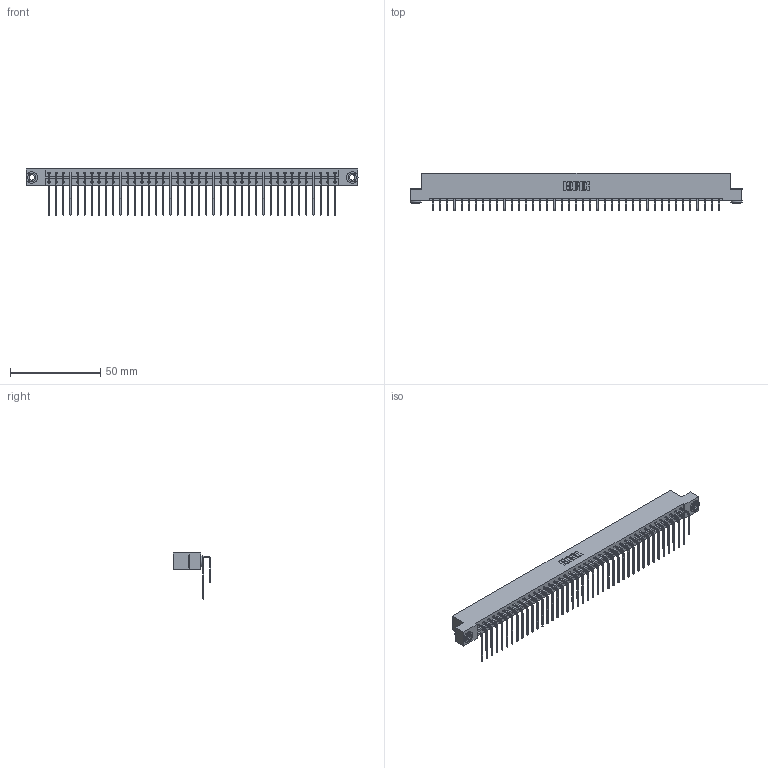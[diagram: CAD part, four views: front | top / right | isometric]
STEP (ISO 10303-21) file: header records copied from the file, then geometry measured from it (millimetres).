
FILE_DESCRIPTION (( 'STEP AP203' ), '1' );
FILE_NAME ('333-082-559-203.STEP', '2018-08-05T03:42:59', ( '' ), ( '' ), 'SwSTEP 2.0', 'SolidWorks 2016', '' );
FILE_SCHEMA (( 'CONFIG_CONTROL_DESIGN' ));
Length unit declared in the file: inch
Products named in the file (5): 345-250-002_345-250-002-102; 333-082-559-203; 333 Part_Flush - .156 Dia - TH; 345-292-001_558 559 Tail - 1; 345-292-001_559 Tail - 2
Assembly tree (85 placements, depth 2):
  333-082-559-203
    333 Part_Flush - .156 Dia - TH
    345-292-001_558 559 Tail - 1  x41
    345-292-001_559 Tail - 2  x41
    345-250-002_345-250-002-102  x2
Bounding box: 184 x 20.9 x 25.53 mm (x, y, z)
Volume: 19268.2 mm3; surface area: 25346.1 mm2
Topology: 85 solids, 85 shells, 4580 faces, 13589 edges, 8946 vertices
Faces by surface type: plane 3196, cylinder 1376, cone 8
Entity records: 28940 total; most frequent: CARTESIAN_POINT 4824, ORIENTED_EDGE 4702, DIRECTION 4137, EDGE_CURVE 2351, LINE 2159, VECTOR 2159, VERTEX_POINT 1562, AXIS2_PLACEMENT_3D 989
